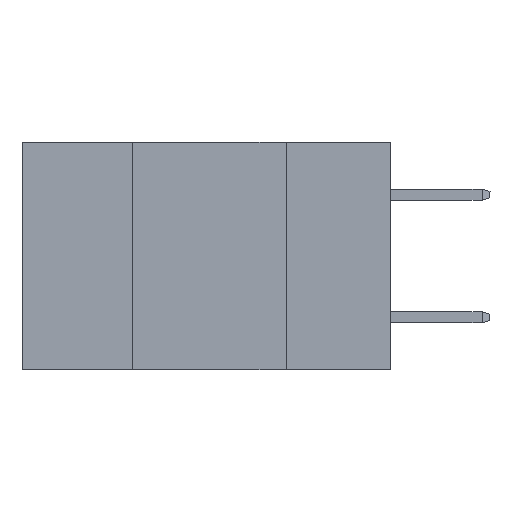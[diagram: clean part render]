
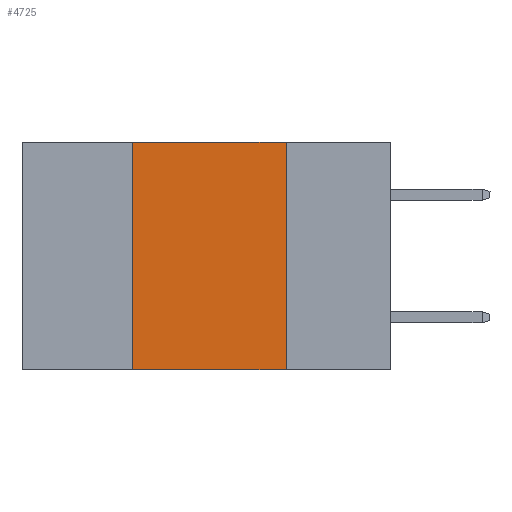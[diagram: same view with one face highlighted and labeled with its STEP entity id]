
A CAD part, left-side view. The second image highlights one B-rep face of the part: STEP entity #4725.
In plain terms, the highlighted planar face has unit normal (-1, 0, 0).
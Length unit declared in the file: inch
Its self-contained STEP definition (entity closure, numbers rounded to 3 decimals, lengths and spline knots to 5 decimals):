
#355 = VECTOR ( 'NONE', #6775, 39.37008 ) ;
#1370 = EDGE_LOOP ( 'NONE', ( #9387, #7908, #10745, #9924 ) ) ;
#1963 = EDGE_CURVE ( 'NONE', #9436, #5422, #7700, .T. ) ;
#2342 = DIRECTION ( 'NONE',  ( 0., 0., -1. ) ) ;
#2785 = LINE ( 'NONE', #4034, #355 ) ;
#2899 = AXIS2_PLACEMENT_3D ( 'NONE', #9878, #9808, #9805 ) ;
#3185 = VERTEX_POINT ( 'NONE', #5199 ) ;
#3325 = CARTESIAN_POINT ( 'NONE',  ( 0., 0.17, 0. ) ) ;
#3737 = CARTESIAN_POINT ( 'NONE',  ( 0., 0.42, 0. ) ) ;
#4034 = CARTESIAN_POINT ( 'NONE',  ( 0., 0.42, 0. ) ) ;
#4725 = ADVANCED_FACE ( 'NONE', ( #8746 ), #9901, .F. ) ;
#5199 = CARTESIAN_POINT ( 'NONE',  ( 0., 0.42, -0.37 ) ) ;
#5382 = VERTEX_POINT ( 'NONE', #3737 ) ;
#5391 = VECTOR ( 'NONE', #2342, 39.37008 ) ;
#5422 = VERTEX_POINT ( 'NONE', #6575 ) ;
#5780 = CARTESIAN_POINT ( 'NONE',  ( 0., 0.17, 0. ) ) ;
#6211 = DIRECTION ( 'NONE',  ( 0., -1., 0. ) ) ;
#6575 = CARTESIAN_POINT ( 'NONE',  ( 0., 0.17, -0.37 ) ) ;
#6775 = DIRECTION ( 'NONE',  ( 0., 0., 1. ) ) ;
#6991 = VECTOR ( 'NONE', #6211, 39.37008 ) ;
#7700 = LINE ( 'NONE', #5780, #5391 ) ;
#7873 = CARTESIAN_POINT ( 'NONE',  ( 0., 0.6, 0. ) ) ;
#7908 = ORIENTED_EDGE ( 'NONE', *, *, #8607, .F. ) ;
#8607 = EDGE_CURVE ( 'NONE', #5382, #9436, #9106, .T. ) ;
#8618 = VECTOR ( 'NONE', #9735, 39.37008 ) ;
#8746 = FACE_OUTER_BOUND ( 'NONE', #1370, .T. ) ;
#9106 = LINE ( 'NONE', #7873, #6991 ) ;
#9203 = EDGE_CURVE ( 'NONE', #3185, #5422, #10683, .T. ) ;
#9387 = ORIENTED_EDGE ( 'NONE', *, *, #1963, .F. ) ;
#9436 = VERTEX_POINT ( 'NONE', #3325 ) ;
#9735 = DIRECTION ( 'NONE',  ( 0., -1., 0. ) ) ;
#9805 = DIRECTION ( 'NONE',  ( 0., 0., -1. ) ) ;
#9808 = DIRECTION ( 'NONE',  ( 1., 0., 0. ) ) ;
#9878 = CARTESIAN_POINT ( 'NONE',  ( 0., 0.6, 0. ) ) ;
#9901 = PLANE ( 'NONE',  #2899 ) ;
#9924 = ORIENTED_EDGE ( 'NONE', *, *, #9203, .T. ) ;
#10208 = EDGE_CURVE ( 'NONE', #3185, #5382, #2785, .T. ) ;
#10485 = CARTESIAN_POINT ( 'NONE',  ( 0., 0.6, -0.37 ) ) ;
#10683 = LINE ( 'NONE', #10485, #8618 ) ;
#10745 = ORIENTED_EDGE ( 'NONE', *, *, #10208, .F. ) ;
